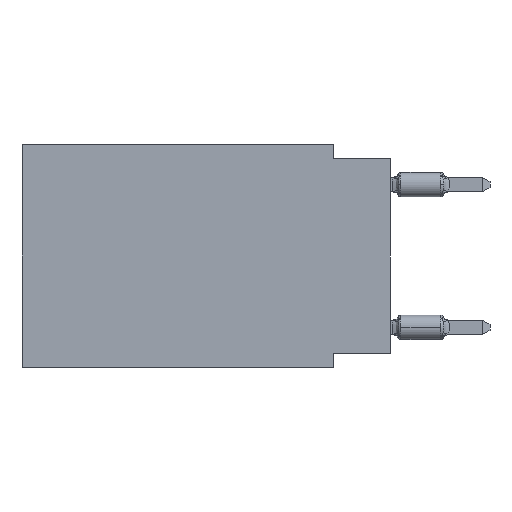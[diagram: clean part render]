
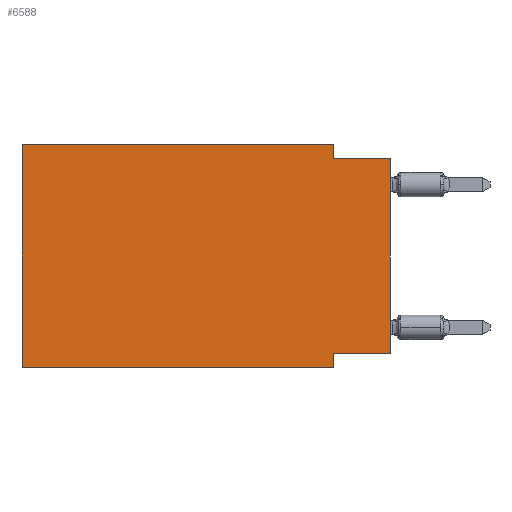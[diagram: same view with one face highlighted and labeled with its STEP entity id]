
A CAD part, left-side view. The second image highlights one B-rep face of the part: STEP entity #6588.
In plain terms, the highlighted planar face has unit normal (-1, 0, 0).
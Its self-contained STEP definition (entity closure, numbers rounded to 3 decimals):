
#47 = VERTEX_POINT ( 'NONE', #7686 ) ;
#472 = CARTESIAN_POINT ( 'NONE',  ( 0., 0., -9.271 ) ) ;
#578 = CARTESIAN_POINT ( 'NONE',  ( 0., 0., -9.271 ) ) ;
#1478 = VECTOR ( 'NONE', #4101, 1000. ) ;
#1532 = LINE ( 'NONE', #7444, #2117 ) ;
#1831 = PLANE ( 'NONE',  #12746 ) ;
#1969 = VECTOR ( 'NONE', #13000, 1000. ) ;
#2117 = VECTOR ( 'NONE', #5459, 1000. ) ;
#2277 = ORIENTED_EDGE ( 'NONE', *, *, #3176, .F. ) ;
#2537 = VERTEX_POINT ( 'NONE', #4573 ) ;
#2798 = LINE ( 'NONE', #13115, #6355 ) ;
#2807 = CARTESIAN_POINT ( 'NONE',  ( 0., 0., -0.635 ) ) ;
#3176 = EDGE_CURVE ( 'NONE', #6301, #47, #9794, .T. ) ;
#3244 = EDGE_CURVE ( 'NONE', #6835, #2537, #9681, .T. ) ;
#3425 = ORIENTED_EDGE ( 'NONE', *, *, #9726, .F. ) ;
#3540 = DIRECTION ( 'NONE',  ( 0., -1., 0. ) ) ;
#3736 = LINE ( 'NONE', #2807, #1969 ) ;
#3739 = CARTESIAN_POINT ( 'NONE',  ( 0., 2.54, -9.906 ) ) ;
#4101 = DIRECTION ( 'NONE',  ( 0., 0., 1. ) ) ;
#4161 = VERTEX_POINT ( 'NONE', #7392 ) ;
#4461 = VECTOR ( 'NONE', #8382, 1000. ) ;
#4573 = CARTESIAN_POINT ( 'NONE',  ( 0., 2.54, -9.271 ) ) ;
#4822 = CARTESIAN_POINT ( 'NONE',  ( 0., 16.383, 0. ) ) ;
#4825 = VECTOR ( 'NONE', #3540, 1000. ) ;
#5338 = VERTEX_POINT ( 'NONE', #10598 ) ;
#5459 = DIRECTION ( 'NONE',  ( 0., -1., 0. ) ) ;
#5501 = EDGE_CURVE ( 'NONE', #47, #4161, #2798, .T. ) ;
#5503 = DIRECTION ( 'NONE',  ( 0., 1., 0. ) ) ;
#5773 = EDGE_CURVE ( 'NONE', #10267, #7488, #1532, .T. ) ;
#5846 = ORIENTED_EDGE ( 'NONE', *, *, #7067, .T. ) ;
#6024 = EDGE_CURVE ( 'NONE', #10267, #6301, #8229, .T. ) ;
#6203 = LINE ( 'NONE', #10455, #4461 ) ;
#6301 = VERTEX_POINT ( 'NONE', #4822 ) ;
#6355 = VECTOR ( 'NONE', #10920, 1000. ) ;
#6588 = ADVANCED_FACE ( 'NONE', ( #8670 ), #1831, .F. ) ;
#6669 = ORIENTED_EDGE ( 'NONE', *, *, #3244, .F. ) ;
#6835 = VERTEX_POINT ( 'NONE', #472 ) ;
#7067 = EDGE_CURVE ( 'NONE', #6835, #5338, #6203, .T. ) ;
#7288 = EDGE_LOOP ( 'NONE', ( #5846, #10224, #11334, #2277, #12673, #9118, #3425, #6669 ) ) ;
#7392 = CARTESIAN_POINT ( 'NONE',  ( 0., 2.54, -0.635 ) ) ;
#7444 = CARTESIAN_POINT ( 'NONE',  ( 0., 16.383, -9.906 ) ) ;
#7488 = VERTEX_POINT ( 'NONE', #12227 ) ;
#7685 = VECTOR ( 'NONE', #5503, 1000. ) ;
#7686 = CARTESIAN_POINT ( 'NONE',  ( 0., 2.54, 0. ) ) ;
#7869 = DIRECTION ( 'NONE',  ( 0., 0., -1. ) ) ;
#8229 = LINE ( 'NONE', #10107, #1478 ) ;
#8293 = CARTESIAN_POINT ( 'NONE',  ( 0., 16.383, -9.906 ) ) ;
#8382 = DIRECTION ( 'NONE',  ( 0., 0., 1. ) ) ;
#8596 = CARTESIAN_POINT ( 'NONE',  ( 0., 16.383, 0. ) ) ;
#8670 = FACE_OUTER_BOUND ( 'NONE', #7288, .T. ) ;
#8724 = LINE ( 'NONE', #3739, #10015 ) ;
#9118 = ORIENTED_EDGE ( 'NONE', *, *, #5773, .T. ) ;
#9681 = LINE ( 'NONE', #578, #7685 ) ;
#9726 = EDGE_CURVE ( 'NONE', #2537, #7488, #8724, .T. ) ;
#9794 = LINE ( 'NONE', #8596, #4825 ) ;
#10015 = VECTOR ( 'NONE', #7869, 1000. ) ;
#10107 = CARTESIAN_POINT ( 'NONE',  ( 0., 16.383, 0. ) ) ;
#10224 = ORIENTED_EDGE ( 'NONE', *, *, #11025, .F. ) ;
#10267 = VERTEX_POINT ( 'NONE', #8293 ) ;
#10455 = CARTESIAN_POINT ( 'NONE',  ( 0., 0., 0. ) ) ;
#10598 = CARTESIAN_POINT ( 'NONE',  ( 0., 0., -0.635 ) ) ;
#10742 = DIRECTION ( 'NONE',  ( 1., 0., 0. ) ) ;
#10920 = DIRECTION ( 'NONE',  ( 0., 0., -1. ) ) ;
#11025 = EDGE_CURVE ( 'NONE', #4161, #5338, #3736, .T. ) ;
#11334 = ORIENTED_EDGE ( 'NONE', *, *, #5501, .F. ) ;
#12227 = CARTESIAN_POINT ( 'NONE',  ( 0., 2.54, -9.906 ) ) ;
#12673 = ORIENTED_EDGE ( 'NONE', *, *, #6024, .F. ) ;
#12734 = CARTESIAN_POINT ( 'NONE',  ( 0., 16.383, 0. ) ) ;
#12746 = AXIS2_PLACEMENT_3D ( 'NONE', #12734, #10742, #12869 ) ;
#12869 = DIRECTION ( 'NONE',  ( 0., 0., -1. ) ) ;
#13000 = DIRECTION ( 'NONE',  ( 0., -1., 0. ) ) ;
#13115 = CARTESIAN_POINT ( 'NONE',  ( 0., 2.54, 0. ) ) ;
